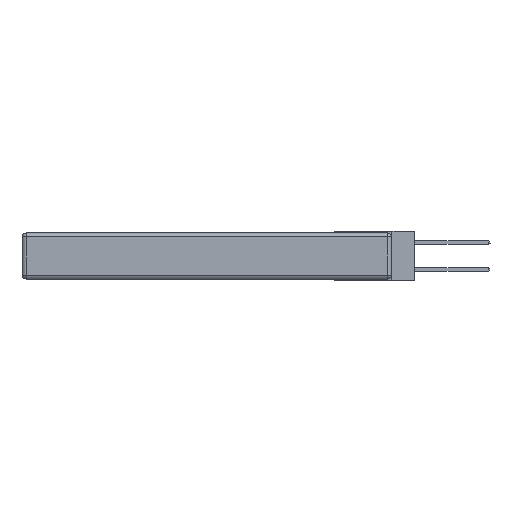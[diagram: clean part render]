
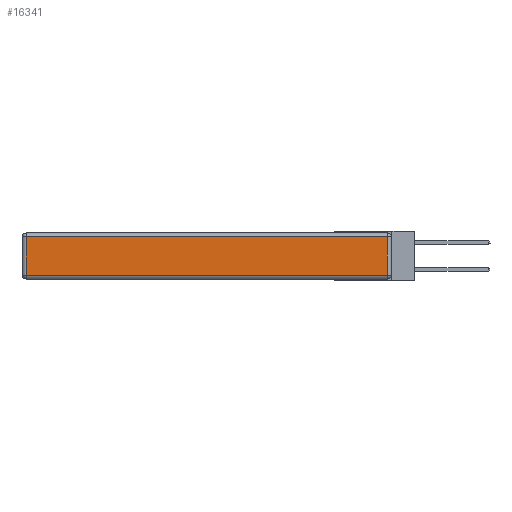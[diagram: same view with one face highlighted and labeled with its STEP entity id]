
A CAD part, left-side view. The second image highlights one B-rep face of the part: STEP entity #16341.
In plain terms, the highlighted planar face has unit normal (-1, 0, 0).
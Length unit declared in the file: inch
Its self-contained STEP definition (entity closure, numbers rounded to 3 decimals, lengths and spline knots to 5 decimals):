
#1082 = PLANE ( 'NONE',  #8825 ) ;
#1473 = DIRECTION ( 'NONE',  ( 0., 0., 1. ) ) ;
#1875 = CARTESIAN_POINT ( 'NONE',  ( 0., 2.72, -0.313 ) ) ;
#2647 = VECTOR ( 'NONE', #1473, 39.37008 ) ;
#2650 = CARTESIAN_POINT ( 'NONE',  ( 0., 0.03, -0.313 ) ) ;
#2873 = VERTEX_POINT ( 'NONE', #4033 ) ;
#3025 = DIRECTION ( 'NONE',  ( 0., 0., -1. ) ) ;
#3185 = ORIENTED_EDGE ( 'NONE', *, *, #14213, .T. ) ;
#3316 = CARTESIAN_POINT ( 'NONE',  ( 0., 0.03, -0.03 ) ) ;
#3537 = CARTESIAN_POINT ( 'NONE',  ( 0., 0., -0.313 ) ) ;
#3997 = EDGE_CURVE ( 'NONE', #5393, #15357, #11296, .T. ) ;
#4033 = CARTESIAN_POINT ( 'NONE',  ( 0., 2.72, -0.03 ) ) ;
#4139 = ORIENTED_EDGE ( 'NONE', *, *, #3997, .T. ) ;
#4727 = CARTESIAN_POINT ( 'NONE',  ( 0., 2.72, -0.343 ) ) ;
#5239 = ORIENTED_EDGE ( 'NONE', *, *, #8683, .T. ) ;
#5393 = VERTEX_POINT ( 'NONE', #2650 ) ;
#7299 = DIRECTION ( 'NONE',  ( 0., 1., 0. ) ) ;
#7363 = CARTESIAN_POINT ( 'NONE',  ( 0., 2.75, -0.03 ) ) ;
#7370 = DIRECTION ( 'NONE',  ( -1., 0., 0. ) ) ;
#7739 = VECTOR ( 'NONE', #7299, 39.37008 ) ;
#8683 = EDGE_CURVE ( 'NONE', #13765, #5393, #9316, .T. ) ;
#8825 = AXIS2_PLACEMENT_3D ( 'NONE', #19663, #7370, #11844 ) ;
#9316 = LINE ( 'NONE', #3537, #16885 ) ;
#10680 = CARTESIAN_POINT ( 'NONE',  ( 0., 0.03, -0.343 ) ) ;
#11296 = LINE ( 'NONE', #10680, #2647 ) ;
#11802 = LINE ( 'NONE', #7363, #7739 ) ;
#11844 = DIRECTION ( 'NONE',  ( 0., 0., 1. ) ) ;
#12802 = DIRECTION ( 'NONE',  ( 0., -1., 0. ) ) ;
#13429 = FACE_OUTER_BOUND ( 'NONE', #19246, .T. ) ;
#13765 = VERTEX_POINT ( 'NONE', #1875 ) ;
#14213 = EDGE_CURVE ( 'NONE', #2873, #13765, #18152, .T. ) ;
#14680 = EDGE_CURVE ( 'NONE', #15357, #2873, #11802, .T. ) ;
#15357 = VERTEX_POINT ( 'NONE', #3316 ) ;
#15923 = ORIENTED_EDGE ( 'NONE', *, *, #14680, .T. ) ;
#16341 = ADVANCED_FACE ( 'NONE', ( #13429 ), #1082, .T. ) ;
#16885 = VECTOR ( 'NONE', #12802, 39.37008 ) ;
#18152 = LINE ( 'NONE', #4727, #18898 ) ;
#18898 = VECTOR ( 'NONE', #3025, 39.37008 ) ;
#19246 = EDGE_LOOP ( 'NONE', ( #5239, #4139, #15923, #3185 ) ) ;
#19663 = CARTESIAN_POINT ( 'NONE',  ( 0., 0., -0.343 ) ) ;
